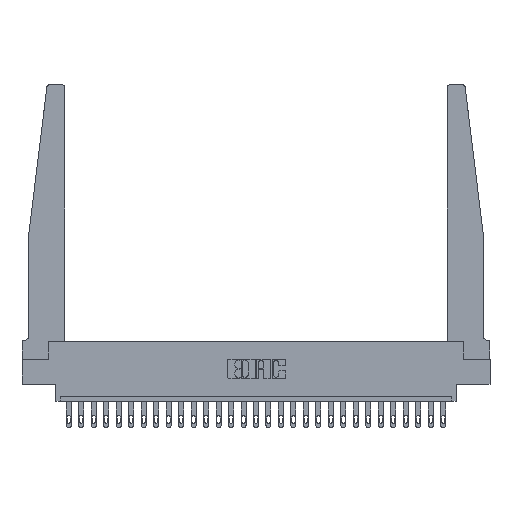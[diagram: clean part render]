
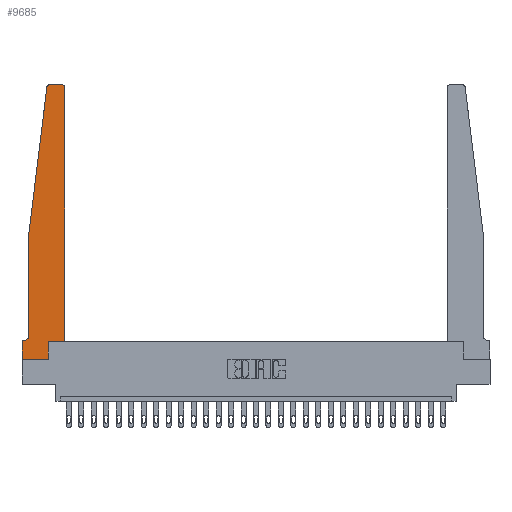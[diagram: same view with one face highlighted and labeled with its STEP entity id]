
A CAD part, top view. The second image highlights one B-rep face of the part: STEP entity #9685.
In plain terms, the highlighted planar face has unit normal (0, 0, 1).
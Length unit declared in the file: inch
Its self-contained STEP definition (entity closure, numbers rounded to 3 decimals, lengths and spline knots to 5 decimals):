
#146 = CARTESIAN_POINT ( 'NONE',  ( 0.065, 1.25, 0.37 ) ) ;
#620 = CARTESIAN_POINT ( 'NONE',  ( 0.065, 1.25, 0.37 ) ) ;
#626 = VERTEX_POINT ( 'NONE', #10839 ) ;
#674 = EDGE_CURVE ( 'NONE', #13663, #22982, #5976, .T. ) ;
#834 = DIRECTION ( 'NONE',  ( 0., -1., 0. ) ) ;
#1248 = CARTESIAN_POINT ( 'NONE',  ( 0., 0., 0.37 ) ) ;
#1271 = CARTESIAN_POINT ( 'NONE',  ( 0., 0.1875, 0.37 ) ) ;
#1335 = EDGE_CURVE ( 'NONE', #13193, #21643, #10689, .T. ) ;
#1343 = ORIENTED_EDGE ( 'NONE', *, *, #15029, .T. ) ;
#1369 = LINE ( 'NONE', #21472, #1825 ) ;
#1825 = VECTOR ( 'NONE', #13319, 39.37008 ) ;
#2065 = VECTOR ( 'NONE', #24807, 39.37008 ) ;
#2104 = PLANE ( 'NONE',  #21558 ) ;
#2813 = CARTESIAN_POINT ( 'NONE',  ( 0.25, 2.75, 0.37 ) ) ;
#2958 = CARTESIAN_POINT ( 'NONE',  ( 0.015, 0.2375, 0.37 ) ) ;
#3023 = EDGE_LOOP ( 'NONE', ( #16380, #6233, #25192, #3769, #18572, #10534, #14367, #19446, #1343, #6286, #21389, #16342 ) ) ;
#3426 = CARTESIAN_POINT ( 'NONE',  ( 0.2605, 0.18, 0.37 ) ) ;
#3510 = DIRECTION ( 'NONE',  ( 0., 0., 1. ) ) ;
#3769 = ORIENTED_EDGE ( 'NONE', *, *, #22149, .T. ) ;
#4116 = VERTEX_POINT ( 'NONE', #12378 ) ;
#4375 = VERTEX_POINT ( 'NONE', #25368 ) ;
#4470 = CARTESIAN_POINT ( 'NONE',  ( 0., 0.1875, 0.37 ) ) ;
#4682 = EDGE_CURVE ( 'NONE', #22982, #18287, #8924, .T. ) ;
#4848 = CARTESIAN_POINT ( 'NONE',  ( 0.425, 0.18, 0.37 ) ) ;
#5270 = AXIS2_PLACEMENT_3D ( 'NONE', #12117, #15940, #10140 ) ;
#5331 = EDGE_CURVE ( 'NONE', #23444, #4375, #22841, .T. ) ;
#5505 = VERTEX_POINT ( 'NONE', #21276 ) ;
#5698 = EDGE_CURVE ( 'NONE', #626, #12521, #22808, .T. ) ;
#5937 = CARTESIAN_POINT ( 'NONE',  ( 0.065, 0.2375, 0.37 ) ) ;
#5976 = CIRCLE ( 'NONE', #20648, 0.05 ) ;
#6057 = FACE_OUTER_BOUND ( 'NONE', #3023, .T. ) ;
#6233 = ORIENTED_EDGE ( 'NONE', *, *, #16225, .T. ) ;
#6286 = ORIENTED_EDGE ( 'NONE', *, *, #5331, .T. ) ;
#6567 = CIRCLE ( 'NONE', #5270, 0.03 ) ;
#7024 = DIRECTION ( 'NONE',  ( -1., 0., 0. ) ) ;
#7223 = VERTEX_POINT ( 'NONE', #15723 ) ;
#7408 = EDGE_CURVE ( 'NONE', #4375, #7223, #1369, .T. ) ;
#7811 = LINE ( 'NONE', #1248, #19802 ) ;
#8404 = DIRECTION ( 'NONE',  ( 1., 0., 0. ) ) ;
#8714 = DIRECTION ( 'NONE',  ( -1., 0., 0. ) ) ;
#8783 = CARTESIAN_POINT ( 'NONE',  ( 0.065, 0.1875, 0.37 ) ) ;
#8924 = LINE ( 'NONE', #8783, #16373 ) ;
#9600 = CARTESIAN_POINT ( 'NONE',  ( 0.015, 0.1875, 0.37 ) ) ;
#9685 = ADVANCED_FACE ( 'NONE', ( #6057 ), #2104, .T. ) ;
#10113 = DIRECTION ( 'NONE',  ( 0., 0., 1. ) ) ;
#10140 = DIRECTION ( 'NONE',  ( 1., 0., 0. ) ) ;
#10435 = CARTESIAN_POINT ( 'NONE',  ( 0.065, 1.25, 0.37 ) ) ;
#10534 = ORIENTED_EDGE ( 'NONE', *, *, #4682, .T. ) ;
#10689 = LINE ( 'NONE', #2813, #13076 ) ;
#10839 = CARTESIAN_POINT ( 'NONE',  ( 0.24675, 2.72367, 0.37 ) ) ;
#11253 = LINE ( 'NONE', #19013, #14961 ) ;
#11621 = DIRECTION ( 'NONE',  ( 1., 0., 0. ) ) ;
#11697 = DIRECTION ( 'NONE',  ( 0., 1., 0. ) ) ;
#12012 = EDGE_CURVE ( 'NONE', #5505, #4116, #7811, .T. ) ;
#12117 = CARTESIAN_POINT ( 'NONE',  ( 0.27653, 2.72, 0.37 ) ) ;
#12378 = CARTESIAN_POINT ( 'NONE',  ( 0.2605, 0., 0.37 ) ) ;
#12521 = VERTEX_POINT ( 'NONE', #146 ) ;
#12597 = DIRECTION ( 'NONE',  ( -1., 0., 0. ) ) ;
#13076 = VECTOR ( 'NONE', #8714, 39.37008 ) ;
#13193 = VERTEX_POINT ( 'NONE', #13986 ) ;
#13319 = DIRECTION ( 'NONE',  ( 0., 1., 0. ) ) ;
#13663 = VERTEX_POINT ( 'NONE', #5937 ) ;
#13986 = CARTESIAN_POINT ( 'NONE',  ( 0.395, 2.75, 0.37 ) ) ;
#14367 = ORIENTED_EDGE ( 'NONE', *, *, #16016, .T. ) ;
#14961 = VECTOR ( 'NONE', #15195, 39.37008 ) ;
#15029 = EDGE_CURVE ( 'NONE', #4116, #23444, #15640, .T. ) ;
#15195 = DIRECTION ( 'NONE',  ( 0., -1., 0. ) ) ;
#15640 = LINE ( 'NONE', #3426, #21652 ) ;
#15723 = CARTESIAN_POINT ( 'NONE',  ( 0.425, 2.72, 0.37 ) ) ;
#15940 = DIRECTION ( 'NONE',  ( 0., 0., 1. ) ) ;
#16001 = CARTESIAN_POINT ( 'NONE',  ( 0.27653, 2.75, 0.37 ) ) ;
#16016 = EDGE_CURVE ( 'NONE', #18287, #5505, #11253, .T. ) ;
#16225 = EDGE_CURVE ( 'NONE', #21643, #626, #6567, .T. ) ;
#16342 = ORIENTED_EDGE ( 'NONE', *, *, #17232, .T. ) ;
#16373 = VECTOR ( 'NONE', #12597, 39.37008 ) ;
#16380 = ORIENTED_EDGE ( 'NONE', *, *, #1335, .T. ) ;
#16629 = AXIS2_PLACEMENT_3D ( 'NONE', #21373, #3510, #19401 ) ;
#17232 = EDGE_CURVE ( 'NONE', #7223, #13193, #21255, .T. ) ;
#18287 = VERTEX_POINT ( 'NONE', #1271 ) ;
#18383 = VECTOR ( 'NONE', #834, 39.37008 ) ;
#18572 = ORIENTED_EDGE ( 'NONE', *, *, #674, .T. ) ;
#19013 = CARTESIAN_POINT ( 'NONE',  ( 0., 0., 0.37 ) ) ;
#19390 = VECTOR ( 'NONE', #24525, 39.37008 ) ;
#19401 = DIRECTION ( 'NONE',  ( 1., 0., 0. ) ) ;
#19446 = ORIENTED_EDGE ( 'NONE', *, *, #12012, .T. ) ;
#19802 = VECTOR ( 'NONE', #11621, 39.37008 ) ;
#20648 = AXIS2_PLACEMENT_3D ( 'NONE', #2958, #25029, #7024 ) ;
#21255 = CIRCLE ( 'NONE', #16629, 0.03 ) ;
#21276 = CARTESIAN_POINT ( 'NONE',  ( 0., 0., 0.37 ) ) ;
#21373 = CARTESIAN_POINT ( 'NONE',  ( 0.395, 2.72, 0.37 ) ) ;
#21389 = ORIENTED_EDGE ( 'NONE', *, *, #7408, .T. ) ;
#21472 = CARTESIAN_POINT ( 'NONE',  ( 0.425, 0.18, 0.37 ) ) ;
#21558 = AXIS2_PLACEMENT_3D ( 'NONE', #4470, #10113, #8404 ) ;
#21643 = VERTEX_POINT ( 'NONE', #16001 ) ;
#21652 = VECTOR ( 'NONE', #11697, 39.37008 ) ;
#22149 = EDGE_CURVE ( 'NONE', #12521, #13663, #22279, .T. ) ;
#22279 = LINE ( 'NONE', #10435, #18383 ) ;
#22808 = LINE ( 'NONE', #620, #19390 ) ;
#22841 = LINE ( 'NONE', #4848, #2065 ) ;
#22912 = CARTESIAN_POINT ( 'NONE',  ( 0.2605, 0.18, 0.37 ) ) ;
#22982 = VERTEX_POINT ( 'NONE', #9600 ) ;
#23444 = VERTEX_POINT ( 'NONE', #22912 ) ;
#24525 = DIRECTION ( 'NONE',  ( -0.122, -0.992, 0. ) ) ;
#24807 = DIRECTION ( 'NONE',  ( 1., 0., 0. ) ) ;
#25029 = DIRECTION ( 'NONE',  ( 0., 0., -1. ) ) ;
#25192 = ORIENTED_EDGE ( 'NONE', *, *, #5698, .T. ) ;
#25368 = CARTESIAN_POINT ( 'NONE',  ( 0.425, 0.18, 0.37 ) ) ;
